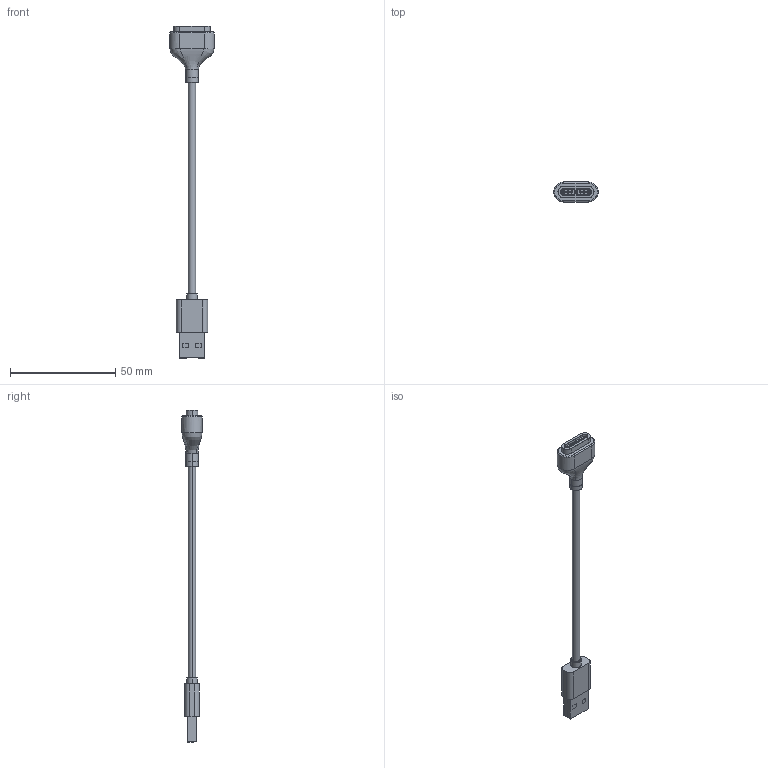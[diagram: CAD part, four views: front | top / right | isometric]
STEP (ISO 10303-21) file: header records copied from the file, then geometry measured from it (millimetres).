
FILE_DESCRIPTION (( 'STEP AP214' ), '1' );
FILE_NAME ('687C0722A101104.STEP', '2023-04-13T15:11:44', ( '' ), ( '' ), 'SwSTEP 2.0', 'SolidWorks 2020', '' );
FILE_SCHEMA (( 'AUTOMOTIVE_DESIGN' ));
Length unit declared in the file: millimetre
Products named in the file (1): 687C0722A101104
Bounding box: 21.1 x 9.5 x 157.4 mm (x, y, z)
Volume: 10860.8 mm3; surface area: 9255.9 mm2
Topology: 2 solids, 22 shells, 550 faces, 1336 edges, 852 vertices
Faces by surface type: plane 242, cylinder 222, torus 30, sphere 28, bspline 14, cone 14
Entity records: 25771 total; most frequent: CARTESIAN_POINT 6499, DIRECTION 2844, ORIENTED_EDGE 2616, EDGE_CURVE 1308, AXIS2_PLACEMENT_3D 1077, VERTEX_POINT 852, LINE 690, VECTOR 690
